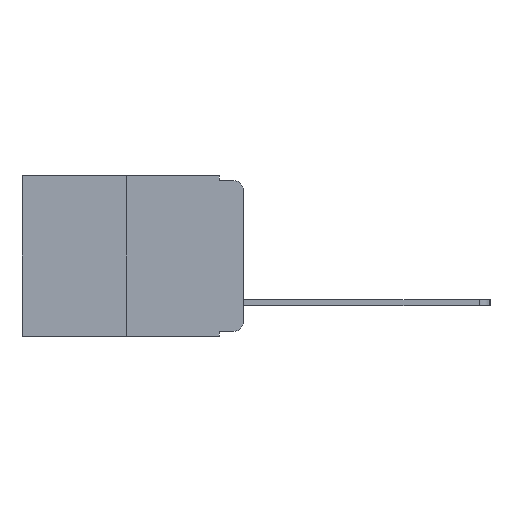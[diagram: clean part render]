
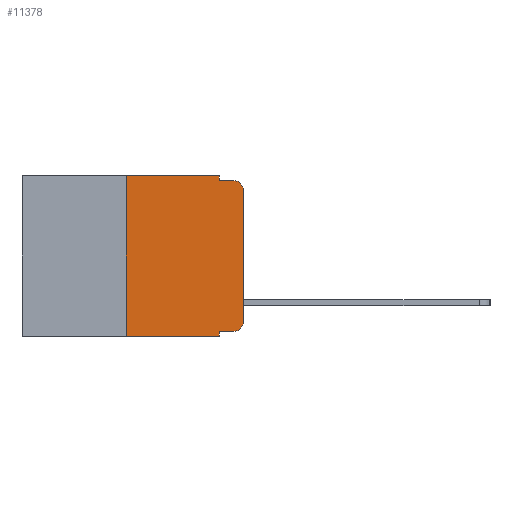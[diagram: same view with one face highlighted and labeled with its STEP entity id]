
A CAD part, left-side view. The second image highlights one B-rep face of the part: STEP entity #11378.
In plain terms, the highlighted planar face has unit normal (-1, 0, 0).
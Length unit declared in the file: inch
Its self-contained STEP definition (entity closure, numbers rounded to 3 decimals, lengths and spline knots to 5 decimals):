
#356 = LINE ( 'NONE', #6251, #8929 ) ;
#465 = EDGE_CURVE ( 'NONE', #3833, #5456, #1414, .T. ) ;
#624 = DIRECTION ( 'NONE',  ( 0., -1., 0. ) ) ;
#822 = VECTOR ( 'NONE', #624, 39.37008 ) ;
#1028 = VECTOR ( 'NONE', #7587, 39.37008 ) ;
#1030 = CARTESIAN_POINT ( 'NONE',  ( 0., 0., -0.03 ) ) ;
#1064 = CARTESIAN_POINT ( 'NONE',  ( 0., 0.02, -0.01 ) ) ;
#1313 = LINE ( 'NONE', #8632, #822 ) ;
#1414 = LINE ( 'NONE', #15376, #1900 ) ;
#1462 = VERTEX_POINT ( 'NONE', #1992 ) ;
#1535 = LINE ( 'NONE', #3475, #10577 ) ;
#1900 = VECTOR ( 'NONE', #4763, 39.37008 ) ;
#1992 = CARTESIAN_POINT ( 'NONE',  ( 0., 0.051, 0. ) ) ;
#2159 = ORIENTED_EDGE ( 'NONE', *, *, #20195, .F. ) ;
#2390 = ORIENTED_EDGE ( 'NONE', *, *, #6535, .F. ) ;
#3002 = ORIENTED_EDGE ( 'NONE', *, *, #17950, .T. ) ;
#3007 = ORIENTED_EDGE ( 'NONE', *, *, #13281, .F. ) ;
#3109 = CARTESIAN_POINT ( 'NONE',  ( 0., 0.25, -0.343 ) ) ;
#3133 = DIRECTION ( 'NONE',  ( 0., -1., 0. ) ) ;
#3380 = CARTESIAN_POINT ( 'NONE',  ( 0., 0., -0.313 ) ) ;
#3475 = CARTESIAN_POINT ( 'NONE',  ( 0., 0.051, 0. ) ) ;
#3833 = VERTEX_POINT ( 'NONE', #11035 ) ;
#4402 = EDGE_CURVE ( 'NONE', #5453, #8501, #5314, .T. ) ;
#4626 = DIRECTION ( 'NONE',  ( 0., 0., 1. ) ) ;
#4763 = DIRECTION ( 'NONE',  ( 0., -1., 0. ) ) ;
#5159 = DIRECTION ( 'NONE',  ( -1., 0., 0. ) ) ;
#5231 = VERTEX_POINT ( 'NONE', #1030 ) ;
#5314 = LINE ( 'NONE', #7639, #1028 ) ;
#5357 = EDGE_LOOP ( 'NONE', ( #3002, #8848, #9879, #2390, #2159, #15640, #17008, #3007, #12022, #5445 ) ) ;
#5376 = AXIS2_PLACEMENT_3D ( 'NONE', #14561, #5159, #16121 ) ;
#5445 = ORIENTED_EDGE ( 'NONE', *, *, #18792, .T. ) ;
#5453 = VERTEX_POINT ( 'NONE', #3109 ) ;
#5456 = VERTEX_POINT ( 'NONE', #9578 ) ;
#5796 = DIRECTION ( 'NONE',  ( 1., 0., 0. ) ) ;
#6251 = CARTESIAN_POINT ( 'NONE',  ( 0., 0., 0. ) ) ;
#6509 = DIRECTION ( 'NONE',  ( -1., 0., 0. ) ) ;
#6530 = VECTOR ( 'NONE', #3133, 39.37008 ) ;
#6535 = EDGE_CURVE ( 'NONE', #1462, #18693, #11103, .T. ) ;
#6731 = DIRECTION ( 'NONE',  ( 0., 0., -1. ) ) ;
#7587 = DIRECTION ( 'NONE',  ( 0., 0., 1. ) ) ;
#7639 = CARTESIAN_POINT ( 'NONE',  ( 0., 0.25, 0. ) ) ;
#8501 = VERTEX_POINT ( 'NONE', #19158 ) ;
#8632 = CARTESIAN_POINT ( 'NONE',  ( 0., 0.473, 0. ) ) ;
#8848 = ORIENTED_EDGE ( 'NONE', *, *, #17044, .T. ) ;
#8929 = VECTOR ( 'NONE', #4626, 39.37008 ) ;
#9279 = DIRECTION ( 'NONE',  ( 0., -1., 0. ) ) ;
#9578 = CARTESIAN_POINT ( 'NONE',  ( 0., 0.02, -0.333 ) ) ;
#9835 = CARTESIAN_POINT ( 'NONE',  ( 0., 0.051, -0.01 ) ) ;
#9879 = ORIENTED_EDGE ( 'NONE', *, *, #14957, .F. ) ;
#10577 = VECTOR ( 'NONE', #6731, 39.37008 ) ;
#10626 = VECTOR ( 'NONE', #18403, 39.37008 ) ;
#10719 = CARTESIAN_POINT ( 'NONE',  ( 0., 0.051, 0. ) ) ;
#11035 = CARTESIAN_POINT ( 'NONE',  ( 0., 0.051, -0.333 ) ) ;
#11103 = LINE ( 'NONE', #10719, #10626 ) ;
#11378 = ADVANCED_FACE ( 'NONE', ( #17639 ), #15184, .F. ) ;
#11553 = LINE ( 'NONE', #18539, #15167 ) ;
#12022 = ORIENTED_EDGE ( 'NONE', *, *, #465, .T. ) ;
#12640 = CIRCLE ( 'NONE', #5376, 0.02 ) ;
#12685 = CARTESIAN_POINT ( 'NONE',  ( 0., 0.051, -0.01 ) ) ;
#12831 = VERTEX_POINT ( 'NONE', #3380 ) ;
#13218 = EDGE_CURVE ( 'NONE', #5453, #14923, #11553, .T. ) ;
#13281 = EDGE_CURVE ( 'NONE', #3833, #14923, #1535, .T. ) ;
#14561 = CARTESIAN_POINT ( 'NONE',  ( 0., 0.02, -0.03 ) ) ;
#14923 = VERTEX_POINT ( 'NONE', #17202 ) ;
#14957 = EDGE_CURVE ( 'NONE', #18693, #19771, #19417, .T. ) ;
#15167 = VECTOR ( 'NONE', #9279, 39.37008 ) ;
#15184 = PLANE ( 'NONE',  #18129 ) ;
#15376 = CARTESIAN_POINT ( 'NONE',  ( 0., 0.051, -0.333 ) ) ;
#15637 = AXIS2_PLACEMENT_3D ( 'NONE', #15880, #6509, #17445 ) ;
#15640 = ORIENTED_EDGE ( 'NONE', *, *, #4402, .F. ) ;
#15880 = CARTESIAN_POINT ( 'NONE',  ( 0., 0.02, -0.313 ) ) ;
#16121 = DIRECTION ( 'NONE',  ( 0., 0., -1. ) ) ;
#16749 = DIRECTION ( 'NONE',  ( 0., 0., -1. ) ) ;
#17008 = ORIENTED_EDGE ( 'NONE', *, *, #13218, .T. ) ;
#17044 = EDGE_CURVE ( 'NONE', #5231, #19771, #12640, .T. ) ;
#17202 = CARTESIAN_POINT ( 'NONE',  ( 0., 0.051, -0.343 ) ) ;
#17445 = DIRECTION ( 'NONE',  ( 0., 0., -1. ) ) ;
#17639 = FACE_OUTER_BOUND ( 'NONE', #5357, .T. ) ;
#17660 = CIRCLE ( 'NONE', #15637, 0.02 ) ;
#17950 = EDGE_CURVE ( 'NONE', #12831, #5231, #356, .T. ) ;
#18129 = AXIS2_PLACEMENT_3D ( 'NONE', #19716, #5796, #16749 ) ;
#18403 = DIRECTION ( 'NONE',  ( 0., 0., -1. ) ) ;
#18539 = CARTESIAN_POINT ( 'NONE',  ( 0., 0.473, -0.343 ) ) ;
#18693 = VERTEX_POINT ( 'NONE', #9835 ) ;
#18792 = EDGE_CURVE ( 'NONE', #5456, #12831, #17660, .T. ) ;
#19158 = CARTESIAN_POINT ( 'NONE',  ( 0., 0.25, 0. ) ) ;
#19417 = LINE ( 'NONE', #12685, #6530 ) ;
#19716 = CARTESIAN_POINT ( 'NONE',  ( 0., 0.473, 0. ) ) ;
#19771 = VERTEX_POINT ( 'NONE', #1064 ) ;
#20195 = EDGE_CURVE ( 'NONE', #8501, #1462, #1313, .T. ) ;
